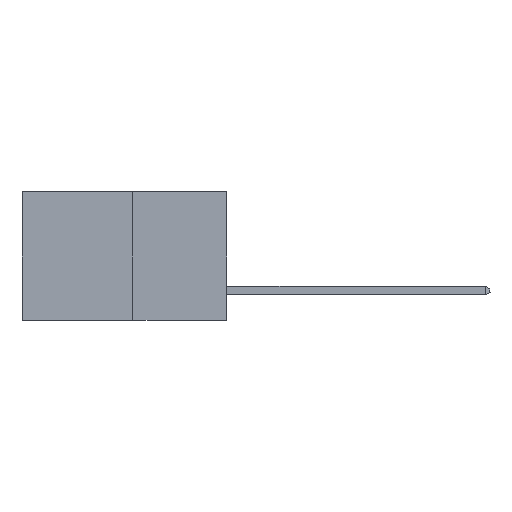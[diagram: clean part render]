
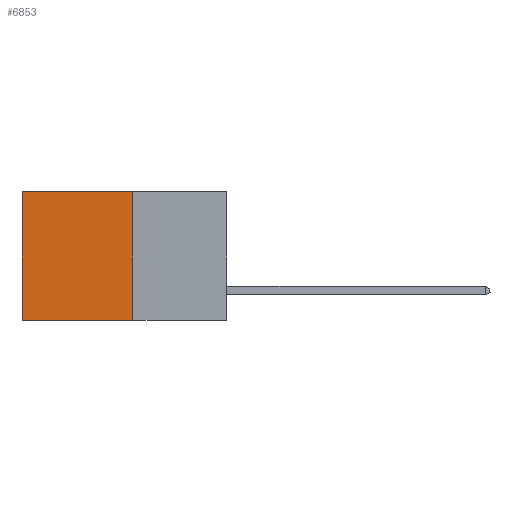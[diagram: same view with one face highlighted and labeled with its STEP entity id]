
A CAD part, left-side view. The second image highlights one B-rep face of the part: STEP entity #6853.
In plain terms, the highlighted planar face has unit normal (-1, 0, 0).
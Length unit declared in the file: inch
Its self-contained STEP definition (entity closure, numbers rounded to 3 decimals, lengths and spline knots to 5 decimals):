
#74 = VECTOR ( 'NONE', #3078, 39.37008 ) ;
#218 = VECTOR ( 'NONE', #4084, 39.37008 ) ;
#304 = ORIENTED_EDGE ( 'NONE', *, *, #19155, .F. ) ;
#2042 = CARTESIAN_POINT ( 'NONE',  ( 0.277, 0.27, -0.37 ) ) ;
#3078 = DIRECTION ( 'NONE',  ( 0., 1., 0. ) ) ;
#3649 = EDGE_LOOP ( 'NONE', ( #26776, #23679, #304, #24114 ) ) ;
#4084 = DIRECTION ( 'NONE',  ( 0., 1., 0. ) ) ;
#5296 = CARTESIAN_POINT ( 'NONE',  ( 0.277, 0.59, -0.37 ) ) ;
#5380 = CARTESIAN_POINT ( 'NONE',  ( 0.277, 0.59, 0. ) ) ;
#6081 = LINE ( 'NONE', #19514, #218 ) ;
#6853 = ADVANCED_FACE ( 'NONE', ( #18260 ), #15280, .F. ) ;
#8126 = VERTEX_POINT ( 'NONE', #27480 ) ;
#9393 = EDGE_CURVE ( 'NONE', #13756, #10774, #18805, .T. ) ;
#9796 = CARTESIAN_POINT ( 'NONE',  ( 0.277, 0.27, 0. ) ) ;
#10774 = VERTEX_POINT ( 'NONE', #5296 ) ;
#13756 = VERTEX_POINT ( 'NONE', #5380 ) ;
#15280 = PLANE ( 'NONE',  #21220 ) ;
#15578 = CARTESIAN_POINT ( 'NONE',  ( 0.277, 0.27, -0.37 ) ) ;
#16104 = DIRECTION ( 'NONE',  ( 0., 0., -1. ) ) ;
#16192 = DIRECTION ( 'NONE',  ( 1., 0., 0. ) ) ;
#16390 = CARTESIAN_POINT ( 'NONE',  ( 0.277, 0.59, -0.37 ) ) ;
#16515 = LINE ( 'NONE', #2042, #21657 ) ;
#17575 = DIRECTION ( 'NONE',  ( 0., 0., -1. ) ) ;
#18093 = VECTOR ( 'NONE', #25321, 39.37008 ) ;
#18260 = FACE_OUTER_BOUND ( 'NONE', #3649, .T. ) ;
#18805 = LINE ( 'NONE', #16390, #18093 ) ;
#19083 = EDGE_CURVE ( 'NONE', #26834, #10774, #6081, .T. ) ;
#19155 = EDGE_CURVE ( 'NONE', #8126, #26834, #16515, .T. ) ;
#19514 = CARTESIAN_POINT ( 'NONE',  ( 0.277, 0.27, -0.37 ) ) ;
#21220 = AXIS2_PLACEMENT_3D ( 'NONE', #15578, #16192, #16104 ) ;
#21657 = VECTOR ( 'NONE', #17575, 39.37008 ) ;
#21943 = EDGE_CURVE ( 'NONE', #8126, #13756, #27472, .T. ) ;
#23611 = CARTESIAN_POINT ( 'NONE',  ( 0.277, 0.27, -0.37 ) ) ;
#23679 = ORIENTED_EDGE ( 'NONE', *, *, #19083, .F. ) ;
#24114 = ORIENTED_EDGE ( 'NONE', *, *, #21943, .T. ) ;
#25321 = DIRECTION ( 'NONE',  ( 0., 0., -1. ) ) ;
#26776 = ORIENTED_EDGE ( 'NONE', *, *, #9393, .T. ) ;
#26834 = VERTEX_POINT ( 'NONE', #23611 ) ;
#27472 = LINE ( 'NONE', #9796, #74 ) ;
#27480 = CARTESIAN_POINT ( 'NONE',  ( 0.277, 0.27, 0. ) ) ;
